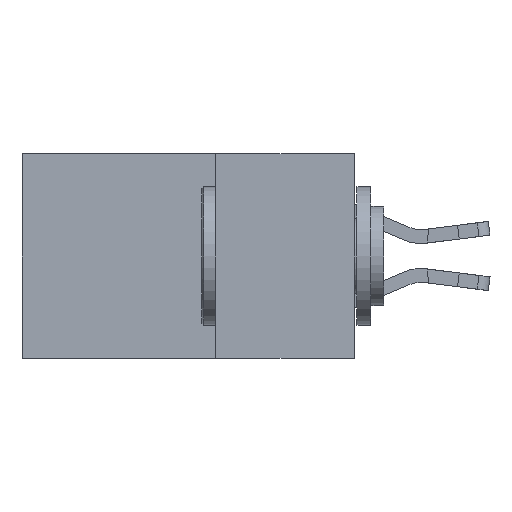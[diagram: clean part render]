
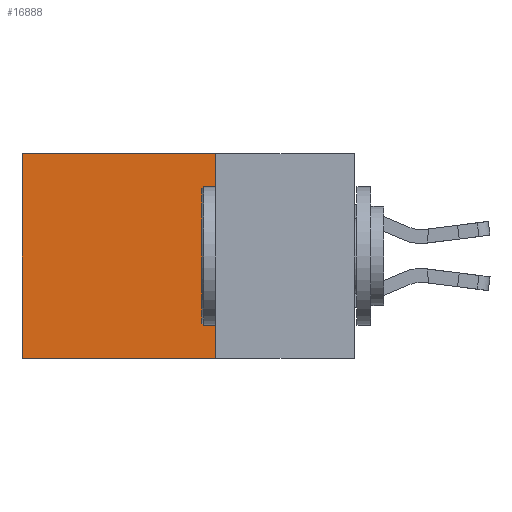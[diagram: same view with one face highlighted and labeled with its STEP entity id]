
A CAD part, left-side view. The second image highlights one B-rep face of the part: STEP entity #16888.
In plain terms, the highlighted planar face has unit normal (-1, 0, 0).
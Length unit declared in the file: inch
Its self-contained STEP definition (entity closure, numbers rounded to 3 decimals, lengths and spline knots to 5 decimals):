
#275 = LINE ( 'NONE', #1239, #7849 ) ;
#728 = DIRECTION ( 'NONE',  ( 0., 0., -1. ) ) ;
#946 = EDGE_CURVE ( 'NONE', #2314, #2190, #11133, .T. ) ;
#1239 = CARTESIAN_POINT ( 'NONE',  ( 0.2615, 0.25, -0.37 ) ) ;
#1438 = PLANE ( 'NONE',  #17037 ) ;
#1904 = FACE_OUTER_BOUND ( 'NONE', #10923, .T. ) ;
#2190 = VERTEX_POINT ( 'NONE', #2992 ) ;
#2314 = VERTEX_POINT ( 'NONE', #9279 ) ;
#2992 = CARTESIAN_POINT ( 'NONE',  ( 0.2615, 0.6, -0.37 ) ) ;
#4000 = ORIENTED_EDGE ( 'NONE', *, *, #946, .T. ) ;
#4496 = DIRECTION ( 'NONE',  ( 1., 0., 0. ) ) ;
#5801 = LINE ( 'NONE', #14180, #17620 ) ;
#6793 = VECTOR ( 'NONE', #728, 39.37008 ) ;
#7112 = CARTESIAN_POINT ( 'NONE',  ( 0.2615, 0.6, -0.37 ) ) ;
#7425 = EDGE_CURVE ( 'NONE', #12787, #2314, #5801, .T. ) ;
#7555 = CARTESIAN_POINT ( 'NONE',  ( 0.2615, 0.25, -0.37 ) ) ;
#7849 = VECTOR ( 'NONE', #11659, 39.37008 ) ;
#9279 = CARTESIAN_POINT ( 'NONE',  ( 0.2615, 0.6, 0. ) ) ;
#10908 = VERTEX_POINT ( 'NONE', #7555 ) ;
#10923 = EDGE_LOOP ( 'NONE', ( #4000, #11405, #17260, #18758 ) ) ;
#11133 = LINE ( 'NONE', #7112, #6793 ) ;
#11405 = ORIENTED_EDGE ( 'NONE', *, *, #16787, .F. ) ;
#11659 = DIRECTION ( 'NONE',  ( 0., 1., 0. ) ) ;
#11996 = CARTESIAN_POINT ( 'NONE',  ( 0.2615, 0.25, 0. ) ) ;
#12787 = VERTEX_POINT ( 'NONE', #11996 ) ;
#13264 = CARTESIAN_POINT ( 'NONE',  ( 0.2615, 0.25, -0.37 ) ) ;
#13945 = CARTESIAN_POINT ( 'NONE',  ( 0.2615, 0.25, -0.37 ) ) ;
#14004 = DIRECTION ( 'NONE',  ( 0., 0., -1. ) ) ;
#14159 = DIRECTION ( 'NONE',  ( 0., 1., 0. ) ) ;
#14180 = CARTESIAN_POINT ( 'NONE',  ( 0.2615, 0.25, 0. ) ) ;
#14685 = DIRECTION ( 'NONE',  ( 0., 0., -1. ) ) ;
#15079 = VECTOR ( 'NONE', #14004, 39.37008 ) ;
#15652 = EDGE_CURVE ( 'NONE', #12787, #10908, #18699, .T. ) ;
#16787 = EDGE_CURVE ( 'NONE', #10908, #2190, #275, .T. ) ;
#16888 = ADVANCED_FACE ( 'NONE', ( #1904 ), #1438, .F. ) ;
#17037 = AXIS2_PLACEMENT_3D ( 'NONE', #13264, #4496, #14685 ) ;
#17260 = ORIENTED_EDGE ( 'NONE', *, *, #15652, .F. ) ;
#17620 = VECTOR ( 'NONE', #14159, 39.37008 ) ;
#18699 = LINE ( 'NONE', #13945, #15079 ) ;
#18758 = ORIENTED_EDGE ( 'NONE', *, *, #7425, .T. ) ;
